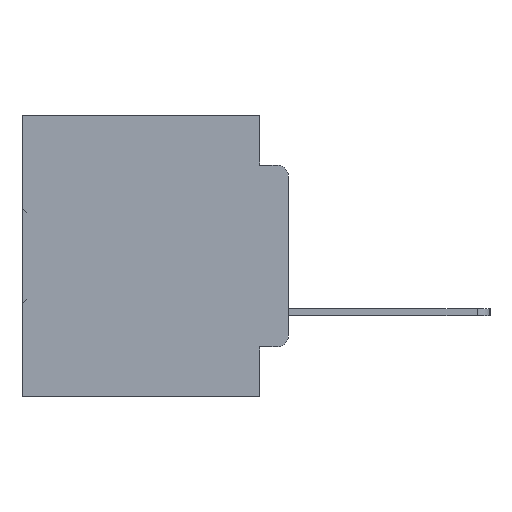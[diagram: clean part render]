
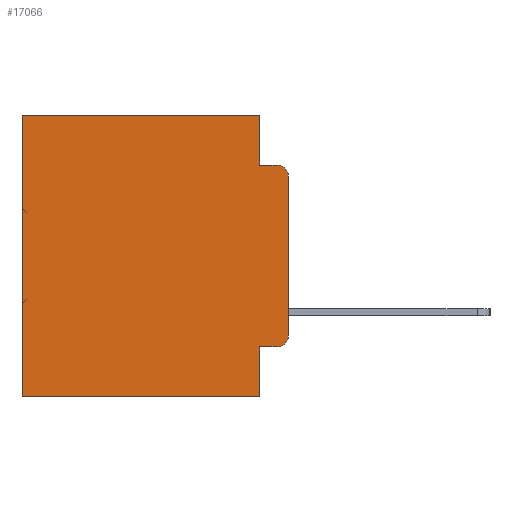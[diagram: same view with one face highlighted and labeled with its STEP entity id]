
A CAD part, left-side view. The second image highlights one B-rep face of the part: STEP entity #17066.
In plain terms, the highlighted planar face has unit normal (-1, 0, 0).
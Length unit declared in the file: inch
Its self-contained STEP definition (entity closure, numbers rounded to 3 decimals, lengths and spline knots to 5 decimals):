
#234 = CIRCLE ( 'NONE', #8624, 0.02 ) ;
#1421 = CARTESIAN_POINT ( 'NONE',  ( 0.298, 0.473, 0. ) ) ;
#1854 = DIRECTION ( 'NONE',  ( -1., 0., 0. ) ) ;
#2881 = CARTESIAN_POINT ( 'NONE',  ( 0.298, 0.051, -0.4115 ) ) ;
#3173 = LINE ( 'NONE', #7763, #23887 ) ;
#4280 = ORIENTED_EDGE ( 'NONE', *, *, #31185, .F. ) ;
#4611 = CARTESIAN_POINT ( 'NONE',  ( 0.298, 0.051, -0.4115 ) ) ;
#4784 = VERTEX_POINT ( 'NONE', #6878 ) ;
#4864 = EDGE_CURVE ( 'NONE', #32823, #24390, #3173, .T. ) ;
#4984 = ORIENTED_EDGE ( 'NONE', *, *, #10603, .T. ) ;
#5029 = ORIENTED_EDGE ( 'NONE', *, *, #18891, .T. ) ;
#6230 = VECTOR ( 'NONE', #18337, 39.37008 ) ;
#6878 = CARTESIAN_POINT ( 'NONE',  ( 0.298, 0., -0.1085 ) ) ;
#7128 = VERTEX_POINT ( 'NONE', #17093 ) ;
#7343 = VECTOR ( 'NONE', #25196, 39.37008 ) ;
#7763 = CARTESIAN_POINT ( 'NONE',  ( 0.298, 0., -0.5 ) ) ;
#8189 = EDGE_CURVE ( 'NONE', #27998, #32823, #14371, .T. ) ;
#8271 = CARTESIAN_POINT ( 'NONE',  ( 0.298, 0.051, -0.0885 ) ) ;
#8624 = AXIS2_PLACEMENT_3D ( 'NONE', #12663, #32062, #15489 ) ;
#9408 = ORIENTED_EDGE ( 'NONE', *, *, #8189, .F. ) ;
#9667 = VECTOR ( 'NONE', #22586, 39.37008 ) ;
#10134 = VECTOR ( 'NONE', #29954, 39.37008 ) ;
#10502 = CARTESIAN_POINT ( 'NONE',  ( 0.298, 0., 0. ) ) ;
#10557 = LINE ( 'NONE', #2881, #9667 ) ;
#10603 = EDGE_CURVE ( 'NONE', #27586, #11921, #234, .T. ) ;
#10775 = VECTOR ( 'NONE', #21272, 39.37008 ) ;
#11554 = FACE_OUTER_BOUND ( 'NONE', #23039, .T. ) ;
#11921 = VERTEX_POINT ( 'NONE', #12940 ) ;
#12663 = CARTESIAN_POINT ( 'NONE',  ( 0.298, 0.02, -0.3915 ) ) ;
#12940 = CARTESIAN_POINT ( 'NONE',  ( 0.298, 0., -0.3915 ) ) ;
#13137 = ORIENTED_EDGE ( 'NONE', *, *, #19972, .F. ) ;
#13746 = CARTESIAN_POINT ( 'NONE',  ( 0.298, 0., 0. ) ) ;
#14371 = LINE ( 'NONE', #27094, #28228 ) ;
#14480 = CARTESIAN_POINT ( 'NONE',  ( 0.298, 0.051, 0. ) ) ;
#15489 = DIRECTION ( 'NONE',  ( 0., 0., -1. ) ) ;
#16565 = AXIS2_PLACEMENT_3D ( 'NONE', #13746, #35879, #19376 ) ;
#17066 = ADVANCED_FACE ( 'NONE', ( #11554 ), #30366, .F. ) ;
#17093 = CARTESIAN_POINT ( 'NONE',  ( 0.298, 0.473, 0. ) ) ;
#17313 = VERTEX_POINT ( 'NONE', #31548 ) ;
#18337 = DIRECTION ( 'NONE',  ( 0., 0., -1. ) ) ;
#18370 = CIRCLE ( 'NONE', #33621, 0.02 ) ;
#18469 = CARTESIAN_POINT ( 'NONE',  ( 0.298, 0.051, 0. ) ) ;
#18560 = ORIENTED_EDGE ( 'NONE', *, *, #4864, .F. ) ;
#18777 = CARTESIAN_POINT ( 'NONE',  ( 0.298, 0.02, -0.1085 ) ) ;
#18864 = CARTESIAN_POINT ( 'NONE',  ( 0.298, 0.051, -0.5 ) ) ;
#18891 = EDGE_CURVE ( 'NONE', #27998, #27586, #10557, .T. ) ;
#19358 = LINE ( 'NONE', #10502, #10134 ) ;
#19376 = DIRECTION ( 'NONE',  ( 0., 0., -1. ) ) ;
#19681 = ORIENTED_EDGE ( 'NONE', *, *, #21881, .T. ) ;
#19972 = EDGE_CURVE ( 'NONE', #17313, #25111, #22292, .T. ) ;
#21272 = DIRECTION ( 'NONE',  ( 0., 0., -1. ) ) ;
#21573 = DIRECTION ( 'NONE',  ( 0., 0., -1. ) ) ;
#21881 = EDGE_CURVE ( 'NONE', #7128, #24390, #34108, .T. ) ;
#22292 = LINE ( 'NONE', #8271, #7343 ) ;
#22475 = CARTESIAN_POINT ( 'NONE',  ( 0.298, 0.02, -0.4115 ) ) ;
#22586 = DIRECTION ( 'NONE',  ( 0., -1., 0. ) ) ;
#23039 = EDGE_LOOP ( 'NONE', ( #34802, #24090, #13137, #4280, #35638, #19681, #18560, #9408, #5029, #4984 ) ) ;
#23887 = VECTOR ( 'NONE', #30076, 39.37008 ) ;
#24090 = ORIENTED_EDGE ( 'NONE', *, *, #24952, .T. ) ;
#24390 = VERTEX_POINT ( 'NONE', #32896 ) ;
#24952 = EDGE_CURVE ( 'NONE', #4784, #25111, #18370, .T. ) ;
#25111 = VERTEX_POINT ( 'NONE', #30468 ) ;
#25196 = DIRECTION ( 'NONE',  ( 0., -1., 0. ) ) ;
#25228 = DIRECTION ( 'NONE',  ( 0., 1., 0. ) ) ;
#25638 = LINE ( 'NONE', #18469, #10775 ) ;
#27094 = CARTESIAN_POINT ( 'NONE',  ( 0.298, 0.051, 0. ) ) ;
#27431 = EDGE_CURVE ( 'NONE', #4784, #11921, #19358, .T. ) ;
#27586 = VERTEX_POINT ( 'NONE', #22475 ) ;
#27926 = CARTESIAN_POINT ( 'NONE',  ( 0.298, 0., 0. ) ) ;
#27998 = VERTEX_POINT ( 'NONE', #4611 ) ;
#28228 = VECTOR ( 'NONE', #30350, 39.37008 ) ;
#28290 = VERTEX_POINT ( 'NONE', #14480 ) ;
#28975 = VECTOR ( 'NONE', #25228, 39.37008 ) ;
#29864 = LINE ( 'NONE', #27926, #28975 ) ;
#29954 = DIRECTION ( 'NONE',  ( 0., 0., -1. ) ) ;
#30076 = DIRECTION ( 'NONE',  ( 0., 1., 0. ) ) ;
#30350 = DIRECTION ( 'NONE',  ( 0., 0., -1. ) ) ;
#30366 = PLANE ( 'NONE',  #16565 ) ;
#30468 = CARTESIAN_POINT ( 'NONE',  ( 0.298, 0.02, -0.0885 ) ) ;
#31185 = EDGE_CURVE ( 'NONE', #28290, #17313, #25638, .T. ) ;
#31548 = CARTESIAN_POINT ( 'NONE',  ( 0.298, 0.051, -0.0885 ) ) ;
#31972 = EDGE_CURVE ( 'NONE', #28290, #7128, #29864, .T. ) ;
#32062 = DIRECTION ( 'NONE',  ( -1., 0., 0. ) ) ;
#32823 = VERTEX_POINT ( 'NONE', #18864 ) ;
#32896 = CARTESIAN_POINT ( 'NONE',  ( 0.298, 0.473, -0.5 ) ) ;
#33621 = AXIS2_PLACEMENT_3D ( 'NONE', #18777, #1854, #21573 ) ;
#34108 = LINE ( 'NONE', #1421, #6230 ) ;
#34802 = ORIENTED_EDGE ( 'NONE', *, *, #27431, .F. ) ;
#35638 = ORIENTED_EDGE ( 'NONE', *, *, #31972, .T. ) ;
#35879 = DIRECTION ( 'NONE',  ( 1., 0., 0. ) ) ;
